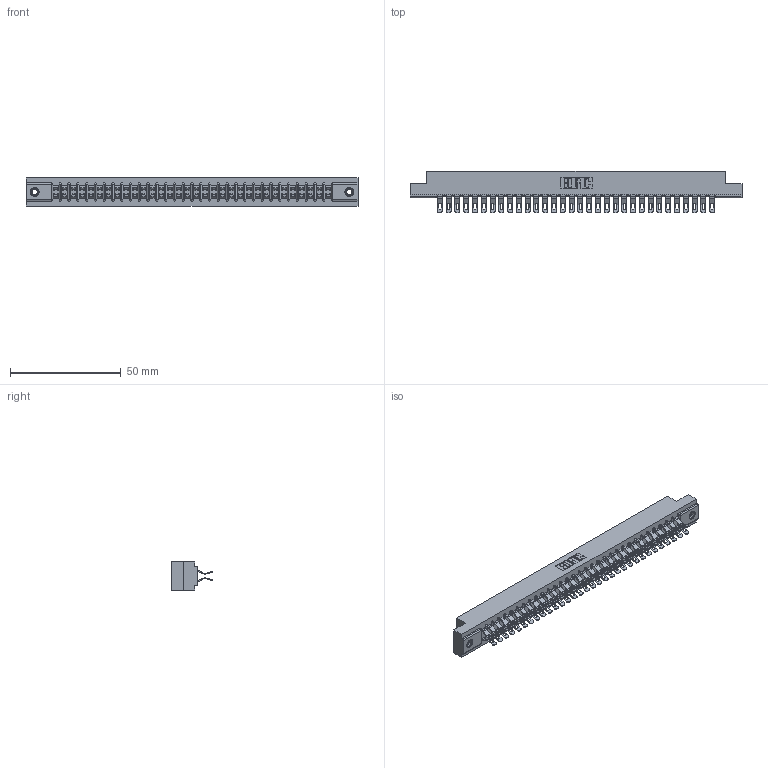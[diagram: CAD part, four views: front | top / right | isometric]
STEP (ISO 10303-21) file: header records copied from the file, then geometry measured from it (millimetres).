
FILE_DESCRIPTION (( 'STEP AP203' ), '1' );
FILE_NAME ('357-064-455-207.STEP', '2020-10-04T17:13:43', ( '' ), ( '' ), 'SwSTEP 2.0', 'SolidWorks 2020', '' );
FILE_SCHEMA (( 'CONFIG_CONTROL_DESIGN' ));
Length unit declared in the file: inch
Products named in the file (4): 307-290-001_555; 345-250-001_345-250-005-103; 307 Part_.156 Dia Mounting Holes; 357-064-455-207
Assembly tree (67 placements, depth 2):
  357-064-455-207
    307 Part_.156 Dia Mounting Holes
    307-290-001_555  x64
    345-250-001_345-250-005-103  x2
Bounding box: 149.81 x 18.75 x 12.7 mm (x, y, z)
Volume: 16036.7 mm3; surface area: 20511.7 mm2
Topology: 67 solids, 67 shells, 4115 faces, 12043 edges, 7846 vertices
Faces by surface type: plane 2278, cylinder 1755, sphere 66, cone 12, torus 4
Entity records: 31412 total; most frequent: CARTESIAN_POINT 5131, ORIENTED_EDGE 5080, DIRECTION 5046, EDGE_CURVE 2540, VECTOR 1932, LINE 1932, VERTEX_POINT 1642, AXIS2_PLACEMENT_3D 1557
